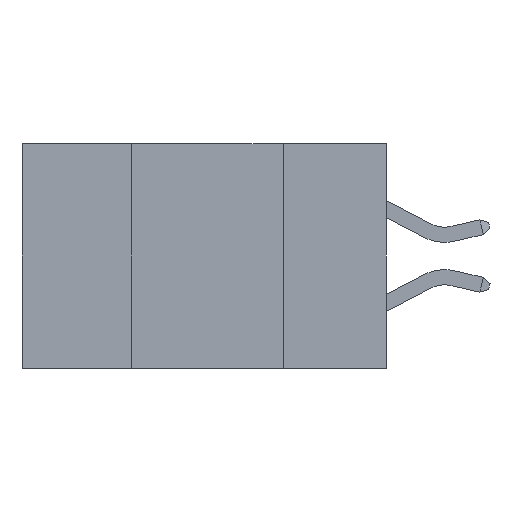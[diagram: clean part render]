
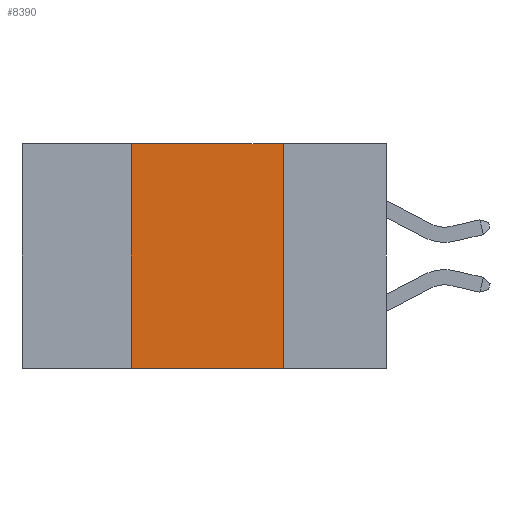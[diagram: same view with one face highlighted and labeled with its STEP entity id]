
A CAD part, left-side view. The second image highlights one B-rep face of the part: STEP entity #8390.
In plain terms, the highlighted planar face has unit normal (-1, 0, 0).
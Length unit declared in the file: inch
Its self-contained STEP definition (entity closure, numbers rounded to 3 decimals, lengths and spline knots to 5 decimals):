
#210 = EDGE_LOOP ( 'NONE', ( #13309, #422, #3554, #4192 ) ) ;
#422 = ORIENTED_EDGE ( 'NONE', *, *, #8199, .F. ) ;
#582 = CARTESIAN_POINT ( 'NONE',  ( 0., 0.6, 0. ) ) ;
#832 = DIRECTION ( 'NONE',  ( 0., -1., 0. ) ) ;
#1115 = CARTESIAN_POINT ( 'NONE',  ( 0., 0.42, -0.37 ) ) ;
#1276 = LINE ( 'NONE', #3396, #9272 ) ;
#1423 = VECTOR ( 'NONE', #9544, 39.37008 ) ;
#1601 = VERTEX_POINT ( 'NONE', #4340 ) ;
#1603 = EDGE_CURVE ( 'NONE', #7949, #1601, #6227, .T. ) ;
#2186 = CARTESIAN_POINT ( 'NONE',  ( 0., 0.17, -0.37 ) ) ;
#3396 = CARTESIAN_POINT ( 'NONE',  ( 0., 0.6, 0. ) ) ;
#3472 = VECTOR ( 'NONE', #6285, 39.37008 ) ;
#3554 = ORIENTED_EDGE ( 'NONE', *, *, #1603, .F. ) ;
#3755 = EDGE_CURVE ( 'NONE', #7949, #4194, #9524, .T. ) ;
#4014 = CARTESIAN_POINT ( 'NONE',  ( 0., 0.17, 0. ) ) ;
#4192 = ORIENTED_EDGE ( 'NONE', *, *, #3755, .T. ) ;
#4194 = VERTEX_POINT ( 'NONE', #2186 ) ;
#4340 = CARTESIAN_POINT ( 'NONE',  ( 0., 0.42, 0. ) ) ;
#5836 = DIRECTION ( 'NONE',  ( 0., 0., -1. ) ) ;
#6075 = CARTESIAN_POINT ( 'NONE',  ( 0., 0.6, -0.37 ) ) ;
#6227 = LINE ( 'NONE', #1115, #3472 ) ;
#6285 = DIRECTION ( 'NONE',  ( 0., 0., 1. ) ) ;
#6418 = VERTEX_POINT ( 'NONE', #4014 ) ;
#6980 = LINE ( 'NONE', #12676, #1423 ) ;
#7949 = VERTEX_POINT ( 'NONE', #11322 ) ;
#8199 = EDGE_CURVE ( 'NONE', #1601, #6418, #1276, .T. ) ;
#8390 = ADVANCED_FACE ( 'NONE', ( #12823 ), #9976, .F. ) ;
#9272 = VECTOR ( 'NONE', #10691, 39.37008 ) ;
#9524 = LINE ( 'NONE', #6075, #12282 ) ;
#9544 = DIRECTION ( 'NONE',  ( 0., 0., -1. ) ) ;
#9976 = PLANE ( 'NONE',  #11945 ) ;
#10232 = EDGE_CURVE ( 'NONE', #6418, #4194, #6980, .T. ) ;
#10691 = DIRECTION ( 'NONE',  ( 0., -1., 0. ) ) ;
#11322 = CARTESIAN_POINT ( 'NONE',  ( 0., 0.42, -0.37 ) ) ;
#11945 = AXIS2_PLACEMENT_3D ( 'NONE', #582, #12055, #5836 ) ;
#12055 = DIRECTION ( 'NONE',  ( 1., 0., 0. ) ) ;
#12282 = VECTOR ( 'NONE', #832, 39.37008 ) ;
#12676 = CARTESIAN_POINT ( 'NONE',  ( 0., 0.17, -0.37 ) ) ;
#12823 = FACE_OUTER_BOUND ( 'NONE', #210, .T. ) ;
#13309 = ORIENTED_EDGE ( 'NONE', *, *, #10232, .F. ) ;
